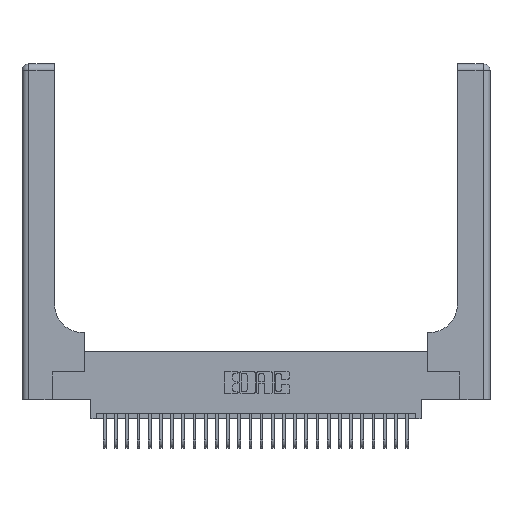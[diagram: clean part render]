
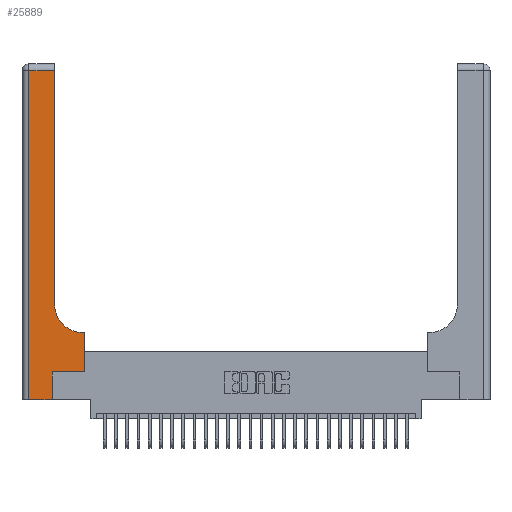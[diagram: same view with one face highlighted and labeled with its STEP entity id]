
A CAD part, top view. The second image highlights one B-rep face of the part: STEP entity #25889.
In plain terms, the highlighted planar face has unit normal (0, 0, 1).
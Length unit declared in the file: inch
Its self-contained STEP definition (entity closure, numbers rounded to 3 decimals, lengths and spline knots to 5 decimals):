
#165 = CARTESIAN_POINT ( 'NONE',  ( 0.5415, 0.85, 0.37 ) ) ;
#1139 = ORIENTED_EDGE ( 'NONE', *, *, #10119, .T. ) ;
#1615 = DIRECTION ( 'NONE',  ( 0., -1., 0. ) ) ;
#2082 = CARTESIAN_POINT ( 'NONE',  ( 0.269, 0.25, 0.37 ) ) ;
#2112 = VERTEX_POINT ( 'NONE', #26414 ) ;
#2480 = ORIENTED_EDGE ( 'NONE', *, *, #19421, .T. ) ;
#2573 = DIRECTION ( 'NONE',  ( 1., 0., 0. ) ) ;
#2974 = CARTESIAN_POINT ( 'NONE',  ( 0.2915, 0.6, 0.37 ) ) ;
#3122 = VERTEX_POINT ( 'NONE', #30211 ) ;
#4064 = CARTESIAN_POINT ( 'NONE',  ( 0.2915, 3., 0.37 ) ) ;
#4201 = AXIS2_PLACEMENT_3D ( 'NONE', #4444, #21106, #6862 ) ;
#4386 = VERTEX_POINT ( 'NONE', #7588 ) ;
#4444 = CARTESIAN_POINT ( 'NONE',  ( 0., 3., 0.37 ) ) ;
#4511 = LINE ( 'NONE', #4064, #16458 ) ;
#4558 = LINE ( 'NONE', #23622, #22807 ) ;
#4712 = CARTESIAN_POINT ( 'NONE',  ( 0.269, 0.25, 0.37 ) ) ;
#4963 = ORIENTED_EDGE ( 'NONE', *, *, #18244, .T. ) ;
#5052 = VERTEX_POINT ( 'NONE', #5151 ) ;
#5151 = CARTESIAN_POINT ( 'NONE',  ( 0.2915, 2.94, 0.37 ) ) ;
#5308 = VECTOR ( 'NONE', #18759, 39.37008 ) ;
#5334 = ORIENTED_EDGE ( 'NONE', *, *, #30730, .T. ) ;
#5748 = VECTOR ( 'NONE', #1615, 39.37008 ) ;
#6003 = LINE ( 'NONE', #29879, #16448 ) ;
#6521 = LINE ( 'NONE', #30126, #5748 ) ;
#6862 = DIRECTION ( 'NONE',  ( -1., 0., 0. ) ) ;
#7187 = VECTOR ( 'NONE', #30500, 39.37008 ) ;
#7588 = CARTESIAN_POINT ( 'NONE',  ( 0.5585, 0.25, 0.37 ) ) ;
#7932 = CIRCLE ( 'NONE', #9281, 0.25 ) ;
#8284 = VECTOR ( 'NONE', #14884, 39.37008 ) ;
#8310 = EDGE_CURVE ( 'NONE', #26804, #5052, #4511, .T. ) ;
#9160 = ORIENTED_EDGE ( 'NONE', *, *, #8310, .T. ) ;
#9281 = AXIS2_PLACEMENT_3D ( 'NONE', #165, #16872, #2573 ) ;
#9394 = DIRECTION ( 'NONE',  ( 0., 1., 0. ) ) ;
#9525 = CARTESIAN_POINT ( 'NONE',  ( 0., 0., 0.37 ) ) ;
#10065 = CARTESIAN_POINT ( 'NONE',  ( 0.06, 2.94, 0.37 ) ) ;
#10119 = EDGE_CURVE ( 'NONE', #5052, #18568, #6003, .T. ) ;
#10270 = VECTOR ( 'NONE', #26136, 39.37008 ) ;
#11992 = CARTESIAN_POINT ( 'NONE',  ( 0.269, 0., 0.37 ) ) ;
#12394 = LINE ( 'NONE', #2082, #5308 ) ;
#13598 = FACE_OUTER_BOUND ( 'NONE', #14778, .T. ) ;
#14262 = LINE ( 'NONE', #25814, #7187 ) ;
#14499 = VERTEX_POINT ( 'NONE', #21553 ) ;
#14778 = EDGE_LOOP ( 'NONE', ( #9160, #1139, #4963, #21247, #30819, #2480, #22566, #5334, #20907 ) ) ;
#14884 = DIRECTION ( 'NONE',  ( -1., 0., 0. ) ) ;
#15155 = EDGE_CURVE ( 'NONE', #4386, #2112, #14262, .T. ) ;
#15204 = CARTESIAN_POINT ( 'NONE',  ( 0.2915, 0.85, 0.37 ) ) ;
#16448 = VECTOR ( 'NONE', #18158, 39.37008 ) ;
#16458 = VECTOR ( 'NONE', #25489, 39.37008 ) ;
#16872 = DIRECTION ( 'NONE',  ( 0., 0., -1. ) ) ;
#16968 = EDGE_CURVE ( 'NONE', #14499, #29877, #28501, .T. ) ;
#18158 = DIRECTION ( 'NONE',  ( -1., 0., 0. ) ) ;
#18244 = EDGE_CURVE ( 'NONE', #18568, #14499, #6521, .T. ) ;
#18568 = VERTEX_POINT ( 'NONE', #10065 ) ;
#18759 = DIRECTION ( 'NONE',  ( 1., 0., 0. ) ) ;
#19421 = EDGE_CURVE ( 'NONE', #29832, #4386, #12394, .T. ) ;
#19466 = EDGE_CURVE ( 'NONE', #29877, #29832, #4558, .T. ) ;
#20907 = ORIENTED_EDGE ( 'NONE', *, *, #30600, .T. ) ;
#21010 = PLANE ( 'NONE',  #4201 ) ;
#21106 = DIRECTION ( 'NONE',  ( 0., 0., -1. ) ) ;
#21247 = ORIENTED_EDGE ( 'NONE', *, *, #16968, .T. ) ;
#21553 = CARTESIAN_POINT ( 'NONE',  ( 0.06, 0., 0.37 ) ) ;
#21706 = LINE ( 'NONE', #2974, #8284 ) ;
#22566 = ORIENTED_EDGE ( 'NONE', *, *, #15155, .T. ) ;
#22807 = VECTOR ( 'NONE', #9394, 39.37008 ) ;
#23622 = CARTESIAN_POINT ( 'NONE',  ( 0.269, 0., 0.37 ) ) ;
#25489 = DIRECTION ( 'NONE',  ( 0., 1., 0. ) ) ;
#25814 = CARTESIAN_POINT ( 'NONE',  ( 0.5585, 0.25, 0.37 ) ) ;
#25889 = ADVANCED_FACE ( 'NONE', ( #13598 ), #21010, .F. ) ;
#26136 = DIRECTION ( 'NONE',  ( 1., 0., 0. ) ) ;
#26414 = CARTESIAN_POINT ( 'NONE',  ( 0.5585, 0.6, 0.37 ) ) ;
#26804 = VERTEX_POINT ( 'NONE', #15204 ) ;
#28501 = LINE ( 'NONE', #9525, #10270 ) ;
#29832 = VERTEX_POINT ( 'NONE', #4712 ) ;
#29877 = VERTEX_POINT ( 'NONE', #11992 ) ;
#29879 = CARTESIAN_POINT ( 'NONE',  ( 0., 2.94, 0.37 ) ) ;
#30126 = CARTESIAN_POINT ( 'NONE',  ( 0.06, 3., 0.37 ) ) ;
#30211 = CARTESIAN_POINT ( 'NONE',  ( 0.5415, 0.6, 0.37 ) ) ;
#30500 = DIRECTION ( 'NONE',  ( 0., 1., 0. ) ) ;
#30600 = EDGE_CURVE ( 'NONE', #3122, #26804, #7932, .T. ) ;
#30730 = EDGE_CURVE ( 'NONE', #2112, #3122, #21706, .T. ) ;
#30819 = ORIENTED_EDGE ( 'NONE', *, *, #19466, .T. ) ;
